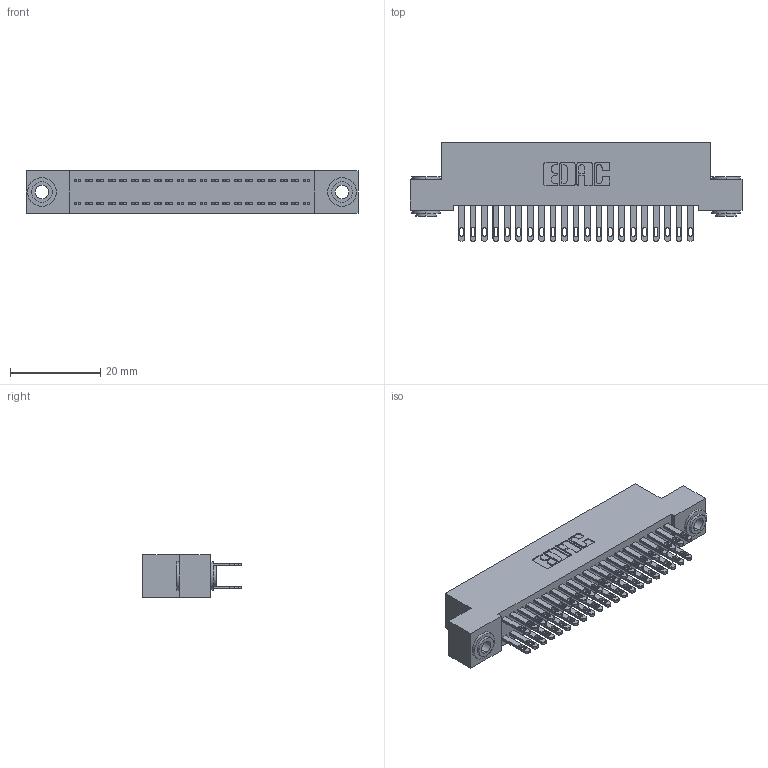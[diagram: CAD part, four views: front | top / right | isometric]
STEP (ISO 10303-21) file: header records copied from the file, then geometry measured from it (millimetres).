
FILE_DESCRIPTION (( 'STEP AP203' ), '1' );
FILE_NAME ('342-042-500-203.STEP', '2018-08-12T02:08:45', ( '' ), ( '' ), 'SwSTEP 2.0', 'SolidWorks 2016', '' );
FILE_SCHEMA (( 'CONFIG_CONTROL_DESIGN' ));
Length unit declared in the file: inch
Products named in the file (4): 342-250-002_345-250-002-102; 342-042-500-203; 342 Part_.156 TH; 345-292-001_345-293-100
Assembly tree (45 placements, depth 2):
  342-042-500-203
    342 Part_.156 TH
    345-292-001_345-293-100  x42
    342-250-002_345-250-002-102  x2
Bounding box: 73.66 x 21.85 x 9.4 mm (x, y, z)
Volume: 6670.1 mm3; surface area: 10956 mm2
Topology: 45 solids, 45 shells, 2164 faces, 6549 edges, 4362 vertices
Faces by surface type: plane 1336, cylinder 820, cone 8
Entity records: 16674 total; most frequent: CARTESIAN_POINT 2761, ORIENTED_EDGE 2690, DIRECTION 2431, EDGE_CURVE 1345, VECTOR 1189, LINE 1189, VERTEX_POINT 894, AXIS2_PLACEMENT_3D 621
